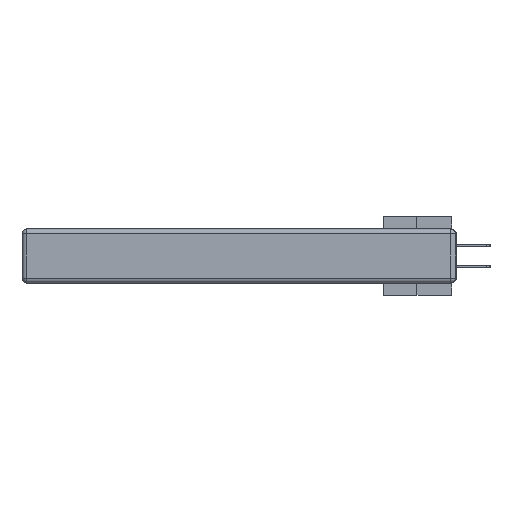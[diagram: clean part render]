
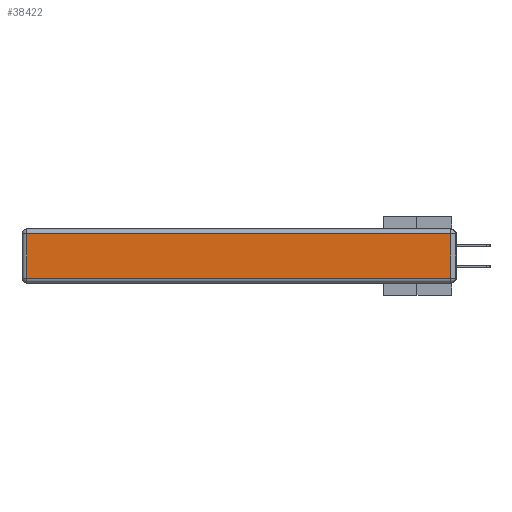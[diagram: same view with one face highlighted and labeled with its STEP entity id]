
A CAD part, left-side view. The second image highlights one B-rep face of the part: STEP entity #38422.
In plain terms, the highlighted planar face has unit normal (-1, 0, 0).
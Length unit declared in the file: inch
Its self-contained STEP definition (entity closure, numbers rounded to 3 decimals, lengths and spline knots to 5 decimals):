
#151 = CARTESIAN_POINT ( 'NONE',  ( 0., 0.03, -0.03 ) ) ;
#701 = DIRECTION ( 'NONE',  ( -1., 0., 0. ) ) ;
#730 = ORIENTED_EDGE ( 'NONE', *, *, #17404, .T. ) ;
#3124 = CARTESIAN_POINT ( 'NONE',  ( 0., 2.72, -0.313 ) ) ;
#3432 = VERTEX_POINT ( 'NONE', #38280 ) ;
#4089 = LINE ( 'NONE', #30940, #11951 ) ;
#4590 = LINE ( 'NONE', #17797, #15518 ) ;
#5332 = LINE ( 'NONE', #5399, #38694 ) ;
#5399 = CARTESIAN_POINT ( 'NONE',  ( 0., 2.75, -0.03 ) ) ;
#5502 = DIRECTION ( 'NONE',  ( 0., 0., 1. ) ) ;
#7459 = CARTESIAN_POINT ( 'NONE',  ( 0., 0., -0.343 ) ) ;
#7777 = DIRECTION ( 'NONE',  ( 0., 0., -1. ) ) ;
#11153 = DIRECTION ( 'NONE',  ( 0., 0., 1. ) ) ;
#11951 = VECTOR ( 'NONE', #7777, 39.37008 ) ;
#14627 = DIRECTION ( 'NONE',  ( 0., -1., 0. ) ) ;
#15518 = VECTOR ( 'NONE', #14627, 39.37008 ) ;
#16419 = LINE ( 'NONE', #20343, #28895 ) ;
#17404 = EDGE_CURVE ( 'NONE', #37017, #29743, #4089, .T. ) ;
#17797 = CARTESIAN_POINT ( 'NONE',  ( 0., 0., -0.313 ) ) ;
#20343 = CARTESIAN_POINT ( 'NONE',  ( 0., 0.03, -0.343 ) ) ;
#21100 = PLANE ( 'NONE',  #33742 ) ;
#26053 = EDGE_CURVE ( 'NONE', #27384, #37017, #5332, .T. ) ;
#26472 = EDGE_CURVE ( 'NONE', #3432, #27384, #16419, .T. ) ;
#27384 = VERTEX_POINT ( 'NONE', #151 ) ;
#28895 = VECTOR ( 'NONE', #5502, 39.37008 ) ;
#29025 = FACE_OUTER_BOUND ( 'NONE', #33053, .T. ) ;
#29743 = VERTEX_POINT ( 'NONE', #3124 ) ;
#30940 = CARTESIAN_POINT ( 'NONE',  ( 0., 2.72, -0.343 ) ) ;
#31499 = ORIENTED_EDGE ( 'NONE', *, *, #26053, .T. ) ;
#31647 = DIRECTION ( 'NONE',  ( 0., 1., 0. ) ) ;
#32121 = CARTESIAN_POINT ( 'NONE',  ( 0., 2.72, -0.03 ) ) ;
#33053 = EDGE_LOOP ( 'NONE', ( #39683, #37821, #31499, #730 ) ) ;
#33742 = AXIS2_PLACEMENT_3D ( 'NONE', #7459, #701, #11153 ) ;
#37017 = VERTEX_POINT ( 'NONE', #32121 ) ;
#37821 = ORIENTED_EDGE ( 'NONE', *, *, #26472, .T. ) ;
#38280 = CARTESIAN_POINT ( 'NONE',  ( 0., 0.03, -0.313 ) ) ;
#38422 = ADVANCED_FACE ( 'NONE', ( #29025 ), #21100, .T. ) ;
#38694 = VECTOR ( 'NONE', #31647, 39.37008 ) ;
#39683 = ORIENTED_EDGE ( 'NONE', *, *, #42912, .T. ) ;
#42912 = EDGE_CURVE ( 'NONE', #29743, #3432, #4590, .T. ) ;
